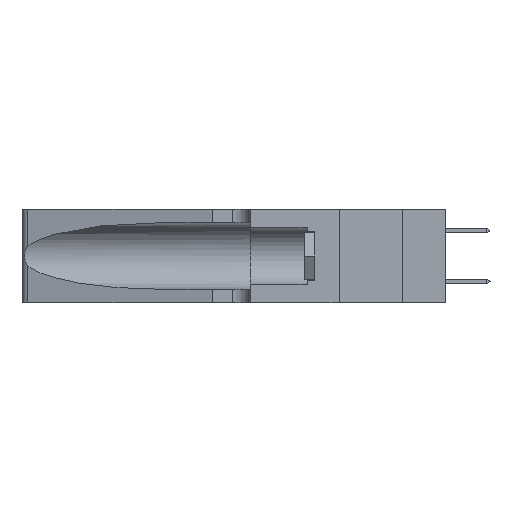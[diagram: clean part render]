
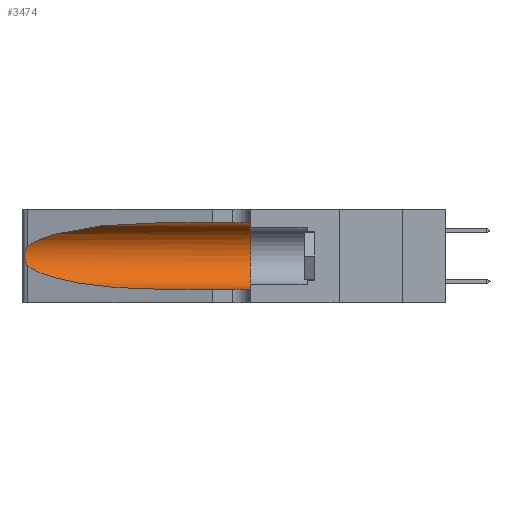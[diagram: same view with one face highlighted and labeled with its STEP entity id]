
A CAD part, left-side view. The second image highlights one B-rep face of the part: STEP entity #3474.
In plain terms, the highlighted cylindrical face has radius 3.308 mm (diameter 6.617 mm), a partial arc.
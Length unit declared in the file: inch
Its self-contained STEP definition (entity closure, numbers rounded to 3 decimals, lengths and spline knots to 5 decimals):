
#76 = VECTOR ( 'NONE', #9548, 39.37008 ) ;
#1000 = CARTESIAN_POINT ( 'NONE',  ( 0.1305, 1.61858, 0.185 ) ) ;
#1218 = ORIENTED_EDGE ( 'NONE', *, *, #2994, .T. ) ;
#1321 = ORIENTED_EDGE ( 'NONE', *, *, #4160, .F. ) ;
#2785 = EDGE_CURVE ( 'NONE', #27758, #9765, #18316, .T. ) ;
#2884 = CARTESIAN_POINT ( 'NONE',  ( 0.18966, 0.96281, 0.05475 ) ) ;
#2888 = LINE ( 'NONE', #22494, #13799 ) ;
#2994 = EDGE_CURVE ( 'NONE', #15122, #12261, #19376, .T. ) ;
#3375 = CARTESIAN_POINT ( 'NONE',  ( 0.25787, 1.23484, 0.2124 ) ) ;
#3474 = ADVANCED_FACE ( 'NONE', ( #12100 ), #3895, .F. ) ;
#3895 = CYLINDRICAL_SURFACE ( 'NONE', #24586, 0.13025 ) ;
#4123 = CARTESIAN_POINT ( 'NONE',  ( 0.18966, 0.96281, 0.31525 ) ) ;
#4160 = EDGE_CURVE ( 'NONE', #18123, #27758, #28066, .T. ) ;
#4914 = DIRECTION ( 'NONE',  ( 0., -1., 0. ) ) ;
#5181 = VERTEX_POINT ( 'NONE', #24801 ) ;
#6434 = ORIENTED_EDGE ( 'NONE', *, *, #2785, .F. ) ;
#6815 = EDGE_LOOP ( 'NONE', ( #13169, #1218, #25870, #7913, #6434, #1321 ) ) ;
#7913 = ORIENTED_EDGE ( 'NONE', *, *, #25278, .T. ) ;
#8726 = CARTESIAN_POINT ( 'NONE',  ( 0.25487, 1.22718, 0.22369 ) ) ;
#8848 = CARTESIAN_POINT ( 'NONE',  ( 0.25789, 1.23486, 0.15765 ) ) ;
#9157 = CARTESIAN_POINT ( 'NONE',  ( 0.2373, 1.15595, 0.08982 ) ) ;
#9319 = CARTESIAN_POINT ( 'NONE',  ( 0.26017, 1.23833, 0.17102 ) ) ;
#9548 = DIRECTION ( 'NONE',  ( 0., -1., 0. ) ) ;
#9622 = CARTESIAN_POINT ( 'NONE',  ( 0.25555, 1.22994, 0.2215 ) ) ;
#9765 = VERTEX_POINT ( 'NONE', #12982 ) ;
#10285 = CARTESIAN_POINT ( 'NONE',  ( 0.25854, 1.2359, 0.20912 ) ) ;
#10705 = CARTESIAN_POINT ( 'NONE',  ( 0.25856, 1.23593, 0.16098 ) ) ;
#11431 = CARTESIAN_POINT ( 'NONE',  ( 0.2373, 1.15595, 0.28018 ) ) ;
#11824 =( BOUNDED_CURVE ( )  B_SPLINE_CURVE ( 3, ( #12896, #4123, #11431, #27520 ),
 .UNSPECIFIED., .F., .T. ) 
 B_SPLINE_CURVE_WITH_KNOTS ( ( 4, 4 ),
 ( 1.5708, 2.84003 ),
 .UNSPECIFIED. ) 
 CURVE ( )  GEOMETRIC_REPRESENTATION_ITEM ( )  RATIONAL_B_SPLINE_CURVE ( ( 1., 0.87, 0.87, 1. ) ) 
 REPRESENTATION_ITEM ( '' )  );
#12100 = FACE_OUTER_BOUND ( 'NONE', #6815, .T. ) ;
#12261 = VERTEX_POINT ( 'NONE', #14554 ) ;
#12896 = CARTESIAN_POINT ( 'NONE',  ( 0.1305, 0.72297, 0.31525 ) ) ;
#12982 = CARTESIAN_POINT ( 'NONE',  ( 0.1305, 0.35, 0.05475 ) ) ;
#13169 = ORIENTED_EDGE ( 'NONE', *, *, #23438, .T. ) ;
#13799 = VECTOR ( 'NONE', #4914, 39.37008 ) ;
#13912 =( BOUNDED_CURVE ( )  B_SPLINE_CURVE ( 3, ( #20081, #9157, #2884, #18175 ),
 .UNSPECIFIED., .F., .F. ) 
 B_SPLINE_CURVE_WITH_KNOTS ( ( 4, 4 ),
 ( 3.44316, 4.71239 ),
 .UNSPECIFIED. ) 
 CURVE ( )  GEOMETRIC_REPRESENTATION_ITEM ( )  RATIONAL_B_SPLINE_CURVE ( ( 1., 0.87, 0.87, 1. ) ) 
 REPRESENTATION_ITEM ( '' )  );
#14554 = CARTESIAN_POINT ( 'NONE',  ( 0.25487, 1.22718, 0.14631 ) ) ;
#15122 = VERTEX_POINT ( 'NONE', #8726 ) ;
#15302 = CARTESIAN_POINT ( 'NONE',  ( 0.25555, 1.22993, 0.14849 ) ) ;
#15580 = DIRECTION ( 'NONE',  ( 0., 1., 0. ) ) ;
#15673 = DIRECTION ( 'NONE',  ( 0., 0., 1. ) ) ;
#15971 = DIRECTION ( 'NONE',  ( 0., -1., 0. ) ) ;
#16202 = CARTESIAN_POINT ( 'NONE',  ( 0.1305, 0.35, 0.31525 ) ) ;
#17470 = CARTESIAN_POINT ( 'NONE',  ( 0.25639, 1.23184, 0.21858 ) ) ;
#17489 = CARTESIAN_POINT ( 'NONE',  ( 0.1305, 0.72297, 0.31525 ) ) ;
#18123 = VERTEX_POINT ( 'NONE', #17489 ) ;
#18175 = CARTESIAN_POINT ( 'NONE',  ( 0.1305, 0.72297, 0.05475 ) ) ;
#18208 = DIRECTION ( 'NONE',  ( 0., 0., -1. ) ) ;
#18316 = CIRCLE ( 'NONE', #24381, 0.13025 ) ;
#18566 = CARTESIAN_POINT ( 'NONE',  ( 0.1305, 1.61858, 0.31525 ) ) ;
#19376 = B_SPLINE_CURVE_WITH_KNOTS ( 'NONE', 3,
 ( #22149, #9622, #17470, #3375, #10285, #21528, #22555, #26885, #9319, #10705, #8848, #19496, #15302, #21616 ),
 .UNSPECIFIED., .F., .F.,
 ( 4, 2, 2, 2, 2, 2, 4 ),
 ( 0., 0.00027, 0.00053, 0.00107, 0.0016, 0.00187, 0.00214 ),
 .UNSPECIFIED. ) ;
#19496 = CARTESIAN_POINT ( 'NONE',  ( 0.25639, 1.23186, 0.15144 ) ) ;
#20081 = CARTESIAN_POINT ( 'NONE',  ( 0.25487, 1.22718, 0.14631 ) ) ;
#20585 = EDGE_CURVE ( 'NONE', #12261, #5181, #13912, .T. ) ;
#21528 = CARTESIAN_POINT ( 'NONE',  ( 0.26018, 1.23835, 0.19895 ) ) ;
#21616 = CARTESIAN_POINT ( 'NONE',  ( 0.25487, 1.22718, 0.14631 ) ) ;
#22149 = CARTESIAN_POINT ( 'NONE',  ( 0.25487, 1.22718, 0.22369 ) ) ;
#22494 = CARTESIAN_POINT ( 'NONE',  ( 0.1305, 1.61858, 0.05475 ) ) ;
#22555 = CARTESIAN_POINT ( 'NONE',  ( 0.26075, 1.23896, 0.19203 ) ) ;
#23438 = EDGE_CURVE ( 'NONE', #18123, #15122, #11824, .T. ) ;
#24381 = AXIS2_PLACEMENT_3D ( 'NONE', #24425, #15580, #15673 ) ;
#24425 = CARTESIAN_POINT ( 'NONE',  ( 0.1305, 0.35, 0.185 ) ) ;
#24586 = AXIS2_PLACEMENT_3D ( 'NONE', #1000, #15971, #18208 ) ;
#24801 = CARTESIAN_POINT ( 'NONE',  ( 0.1305, 0.72297, 0.05475 ) ) ;
#25278 = EDGE_CURVE ( 'NONE', #5181, #9765, #2888, .T. ) ;
#25870 = ORIENTED_EDGE ( 'NONE', *, *, #20585, .T. ) ;
#26885 = CARTESIAN_POINT ( 'NONE',  ( 0.26075, 1.23896, 0.178 ) ) ;
#27520 = CARTESIAN_POINT ( 'NONE',  ( 0.25487, 1.22718, 0.22369 ) ) ;
#27758 = VERTEX_POINT ( 'NONE', #16202 ) ;
#28066 = LINE ( 'NONE', #18566, #76 ) ;
